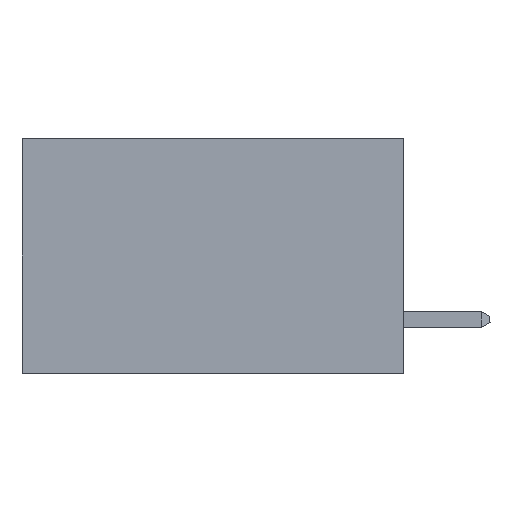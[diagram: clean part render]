
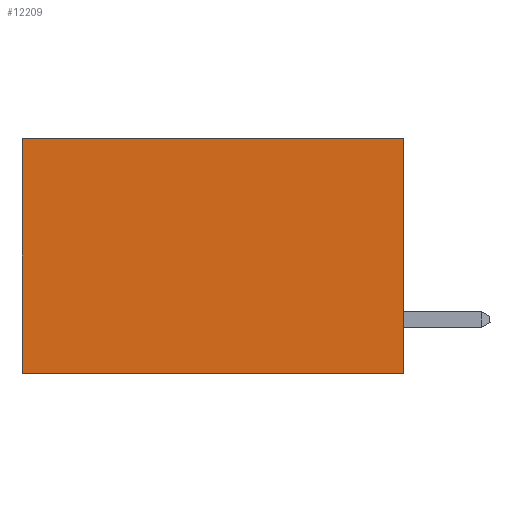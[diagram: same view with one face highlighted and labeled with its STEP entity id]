
A CAD part, left-side view. The second image highlights one B-rep face of the part: STEP entity #12209.
In plain terms, the highlighted planar face has unit normal (-1, 0, 0).
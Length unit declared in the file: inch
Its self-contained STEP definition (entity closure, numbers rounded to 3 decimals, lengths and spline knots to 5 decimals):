
#5 = EDGE_CURVE ( 'NONE', #12769, #17003, #12771, .T. ) ;
#1251 = CARTESIAN_POINT ( 'NONE',  ( 0.2875, 0.6, -0.37 ) ) ;
#1871 = CARTESIAN_POINT ( 'NONE',  ( 0.2875, 0., -0.37 ) ) ;
#2023 = EDGE_CURVE ( 'NONE', #7877, #17003, #12688, .T. ) ;
#2360 = VECTOR ( 'NONE', #12566, 39.37008 ) ;
#2686 = ORIENTED_EDGE ( 'NONE', *, *, #13607, .T. ) ;
#2737 = CARTESIAN_POINT ( 'NONE',  ( 0.2875, 0., -0.37 ) ) ;
#2772 = ORIENTED_EDGE ( 'NONE', *, *, #16186, .F. ) ;
#5348 = DIRECTION ( 'NONE',  ( 0., 0., -1. ) ) ;
#7275 = CARTESIAN_POINT ( 'NONE',  ( 0.2875, 0., 0. ) ) ;
#7714 = FACE_OUTER_BOUND ( 'NONE', #21615, .T. ) ;
#7877 = VERTEX_POINT ( 'NONE', #11559 ) ;
#7961 = VECTOR ( 'NONE', #8386, 39.37008 ) ;
#8386 = DIRECTION ( 'NONE',  ( 0., 0., -1. ) ) ;
#8495 = DIRECTION ( 'NONE',  ( 0., 0., -1. ) ) ;
#8666 = VECTOR ( 'NONE', #5348, 39.37008 ) ;
#8830 = ORIENTED_EDGE ( 'NONE', *, *, #5, .F. ) ;
#9774 = LINE ( 'NONE', #23105, #8666 ) ;
#10613 = VERTEX_POINT ( 'NONE', #22736 ) ;
#11559 = CARTESIAN_POINT ( 'NONE',  ( 0.2875, 0.6, 0. ) ) ;
#12209 = ADVANCED_FACE ( 'NONE', ( #7714 ), #22583, .F. ) ;
#12566 = DIRECTION ( 'NONE',  ( 0., 1., 0. ) ) ;
#12688 = LINE ( 'NONE', #17531, #7961 ) ;
#12769 = VERTEX_POINT ( 'NONE', #2737 ) ;
#12771 = LINE ( 'NONE', #1871, #2360 ) ;
#13270 = LINE ( 'NONE', #7275, #19993 ) ;
#13607 = EDGE_CURVE ( 'NONE', #10613, #7877, #13270, .T. ) ;
#13754 = ORIENTED_EDGE ( 'NONE', *, *, #2023, .T. ) ;
#15091 = AXIS2_PLACEMENT_3D ( 'NONE', #15605, #17258, #8495 ) ;
#15605 = CARTESIAN_POINT ( 'NONE',  ( 0.2875, 0., 0. ) ) ;
#16186 = EDGE_CURVE ( 'NONE', #10613, #12769, #9774, .T. ) ;
#17003 = VERTEX_POINT ( 'NONE', #1251 ) ;
#17258 = DIRECTION ( 'NONE',  ( 1., 0., 0. ) ) ;
#17531 = CARTESIAN_POINT ( 'NONE',  ( 0.2875, 0.6, 0. ) ) ;
#18256 = DIRECTION ( 'NONE',  ( 0., 1., 0. ) ) ;
#19993 = VECTOR ( 'NONE', #18256, 39.37008 ) ;
#21615 = EDGE_LOOP ( 'NONE', ( #13754, #8830, #2772, #2686 ) ) ;
#22583 = PLANE ( 'NONE',  #15091 ) ;
#22736 = CARTESIAN_POINT ( 'NONE',  ( 0.2875, 0., 0. ) ) ;
#23105 = CARTESIAN_POINT ( 'NONE',  ( 0.2875, 0., 0. ) ) ;
